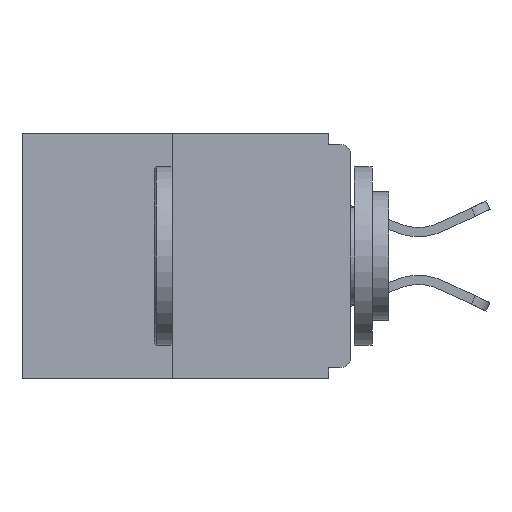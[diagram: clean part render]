
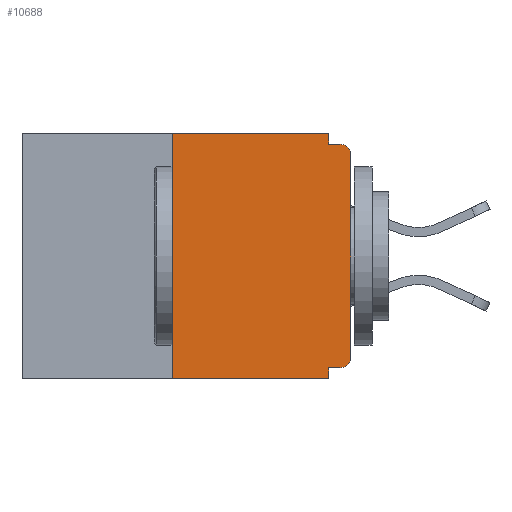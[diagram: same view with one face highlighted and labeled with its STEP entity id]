
A CAD part, left-side view. The second image highlights one B-rep face of the part: STEP entity #10688.
In plain terms, the highlighted planar face has unit normal (-1, 0, 0).
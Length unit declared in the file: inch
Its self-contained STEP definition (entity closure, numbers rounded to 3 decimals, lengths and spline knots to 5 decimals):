
#49 = AXIS2_PLACEMENT_3D ( 'NONE', #18110, #14791, #7555 ) ;
#144 = CARTESIAN_POINT ( 'NONE',  ( 0., 0.015, -0.015 ) ) ;
#427 = DIRECTION ( 'NONE',  ( 0., -1., 0. ) ) ;
#433 = CARTESIAN_POINT ( 'NONE',  ( 0., 0., 0. ) ) ;
#1169 = VERTEX_POINT ( 'NONE', #15685 ) ;
#1213 = DIRECTION ( 'NONE',  ( 0., -1., 0. ) ) ;
#1447 = LINE ( 'NONE', #6091, #12982 ) ;
#1466 = CARTESIAN_POINT ( 'NONE',  ( 0., 0.031, -0.343 ) ) ;
#1632 = VECTOR ( 'NONE', #14728, 39.37008 ) ;
#1983 = VECTOR ( 'NONE', #19709, 39.37008 ) ;
#2663 = EDGE_CURVE ( 'NONE', #8184, #17461, #22708, .T. ) ;
#2776 = DIRECTION ( 'NONE',  ( 0., 0., -1. ) ) ;
#2797 = EDGE_CURVE ( 'NONE', #6208, #1169, #8614, .T. ) ;
#3560 = ORIENTED_EDGE ( 'NONE', *, *, #4590, .F. ) ;
#4045 = ORIENTED_EDGE ( 'NONE', *, *, #10787, .T. ) ;
#4077 = ORIENTED_EDGE ( 'NONE', *, *, #9867, .T. ) ;
#4207 = DIRECTION ( 'NONE',  ( 1., 0., 0. ) ) ;
#4378 = EDGE_CURVE ( 'NONE', #17461, #11383, #1447, .T. ) ;
#4439 = LINE ( 'NONE', #7977, #1983 ) ;
#4483 = DIRECTION ( 'NONE',  ( 0., 0., -1. ) ) ;
#4525 = FACE_OUTER_BOUND ( 'NONE', #6792, .T. ) ;
#4590 = EDGE_CURVE ( 'NONE', #10948, #7909, #4439, .T. ) ;
#5869 = DIRECTION ( 'NONE',  ( 0., -1., 0. ) ) ;
#6091 = CARTESIAN_POINT ( 'NONE',  ( 0., 0., -0.015 ) ) ;
#6208 = VERTEX_POINT ( 'NONE', #16308 ) ;
#6792 = EDGE_LOOP ( 'NONE', ( #7733, #3560, #4077, #16143, #18884, #9336, #17402, #4045, #13521, #7040 ) ) ;
#6830 = EDGE_CURVE ( 'NONE', #13178, #6208, #19507, .T. ) ;
#7040 = ORIENTED_EDGE ( 'NONE', *, *, #2663, .F. ) ;
#7069 = CARTESIAN_POINT ( 'NONE',  ( 0., 0.25, -0.343 ) ) ;
#7555 = DIRECTION ( 'NONE',  ( 0., 0., -1. ) ) ;
#7626 = CARTESIAN_POINT ( 'NONE',  ( 0., 0.46, 0. ) ) ;
#7733 = ORIENTED_EDGE ( 'NONE', *, *, #14608, .F. ) ;
#7909 = VERTEX_POINT ( 'NONE', #15745 ) ;
#7977 = CARTESIAN_POINT ( 'NONE',  ( 0., 0.25, 0. ) ) ;
#8184 = VERTEX_POINT ( 'NONE', #14419 ) ;
#8523 = EDGE_CURVE ( 'NONE', #20740, #17863, #12806, .T. ) ;
#8614 = LINE ( 'NONE', #1466, #17479 ) ;
#8676 = PLANE ( 'NONE',  #15765 ) ;
#8720 = LINE ( 'NONE', #14360, #12333 ) ;
#9336 = ORIENTED_EDGE ( 'NONE', *, *, #13653, .T. ) ;
#9753 = VECTOR ( 'NONE', #1213, 39.37008 ) ;
#9867 = EDGE_CURVE ( 'NONE', #10948, #1169, #14183, .T. ) ;
#9996 = CIRCLE ( 'NONE', #49, 0.015 ) ;
#10688 = ADVANCED_FACE ( 'NONE', ( #4525 ), #8676, .F. ) ;
#10787 = EDGE_CURVE ( 'NONE', #17863, #11383, #9996, .T. ) ;
#10948 = VERTEX_POINT ( 'NONE', #7069 ) ;
#11383 = VERTEX_POINT ( 'NONE', #144 ) ;
#11515 = DIRECTION ( 'NONE',  ( -1., 0., 0. ) ) ;
#12333 = VECTOR ( 'NONE', #427, 39.37008 ) ;
#12646 = CARTESIAN_POINT ( 'NONE',  ( 0., 0., -0.328 ) ) ;
#12806 = LINE ( 'NONE', #433, #13898 ) ;
#12982 = VECTOR ( 'NONE', #5869, 39.37008 ) ;
#13178 = VERTEX_POINT ( 'NONE', #18899 ) ;
#13263 = CARTESIAN_POINT ( 'NONE',  ( 0., 0.031, 0. ) ) ;
#13300 = CARTESIAN_POINT ( 'NONE',  ( 0., 0., -0.03 ) ) ;
#13407 = CARTESIAN_POINT ( 'NONE',  ( 0., 0., -0.313 ) ) ;
#13521 = ORIENTED_EDGE ( 'NONE', *, *, #4378, .F. ) ;
#13653 = EDGE_CURVE ( 'NONE', #13178, #20740, #22590, .T. ) ;
#13875 = DIRECTION ( 'NONE',  ( 0., 0., -1. ) ) ;
#13898 = VECTOR ( 'NONE', #21546, 39.37008 ) ;
#14183 = LINE ( 'NONE', #16940, #9753 ) ;
#14360 = CARTESIAN_POINT ( 'NONE',  ( 0., 0.46, 0. ) ) ;
#14419 = CARTESIAN_POINT ( 'NONE',  ( 0., 0.031, 0. ) ) ;
#14608 = EDGE_CURVE ( 'NONE', #7909, #8184, #8720, .T. ) ;
#14728 = DIRECTION ( 'NONE',  ( 0., 1., 0. ) ) ;
#14791 = DIRECTION ( 'NONE',  ( -1., 0., 0. ) ) ;
#15224 = CARTESIAN_POINT ( 'NONE',  ( 0., 0.015, -0.313 ) ) ;
#15685 = CARTESIAN_POINT ( 'NONE',  ( 0., 0.031, -0.343 ) ) ;
#15745 = CARTESIAN_POINT ( 'NONE',  ( 0., 0.25, 0. ) ) ;
#15765 = AXIS2_PLACEMENT_3D ( 'NONE', #7626, #4207, #16648 ) ;
#16143 = ORIENTED_EDGE ( 'NONE', *, *, #2797, .F. ) ;
#16308 = CARTESIAN_POINT ( 'NONE',  ( 0., 0.031, -0.328 ) ) ;
#16648 = DIRECTION ( 'NONE',  ( 0., 0., -1. ) ) ;
#16940 = CARTESIAN_POINT ( 'NONE',  ( 0., 0.46, -0.343 ) ) ;
#16969 = AXIS2_PLACEMENT_3D ( 'NONE', #15224, #11515, #4483 ) ;
#17402 = ORIENTED_EDGE ( 'NONE', *, *, #8523, .T. ) ;
#17461 = VERTEX_POINT ( 'NONE', #19238 ) ;
#17479 = VECTOR ( 'NONE', #13875, 39.37008 ) ;
#17863 = VERTEX_POINT ( 'NONE', #13300 ) ;
#18032 = VECTOR ( 'NONE', #2776, 39.37008 ) ;
#18110 = CARTESIAN_POINT ( 'NONE',  ( 0., 0.015, -0.03 ) ) ;
#18884 = ORIENTED_EDGE ( 'NONE', *, *, #6830, .F. ) ;
#18899 = CARTESIAN_POINT ( 'NONE',  ( 0., 0.015, -0.328 ) ) ;
#19238 = CARTESIAN_POINT ( 'NONE',  ( 0., 0.031, -0.015 ) ) ;
#19507 = LINE ( 'NONE', #12646, #1632 ) ;
#19709 = DIRECTION ( 'NONE',  ( 0., 0., 1. ) ) ;
#20740 = VERTEX_POINT ( 'NONE', #13407 ) ;
#21546 = DIRECTION ( 'NONE',  ( 0., 0., 1. ) ) ;
#22590 = CIRCLE ( 'NONE', #16969, 0.015 ) ;
#22708 = LINE ( 'NONE', #13263, #18032 ) ;
